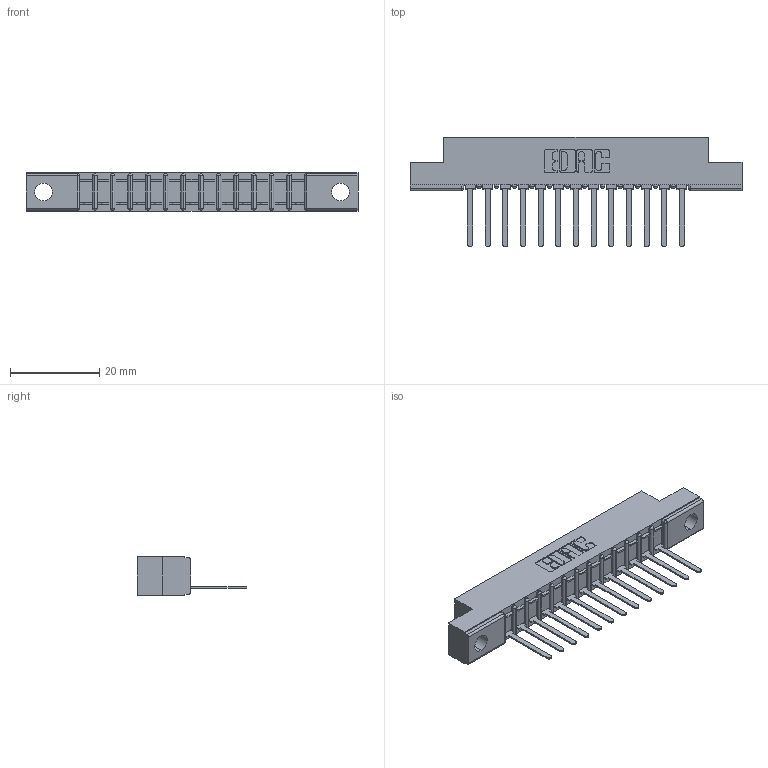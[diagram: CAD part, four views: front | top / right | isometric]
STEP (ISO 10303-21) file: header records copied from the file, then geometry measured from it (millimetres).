
FILE_DESCRIPTION (( 'STEP AP203' ), '1' );
FILE_NAME ('307-013-541-102.STEP', '2019-09-04T20:11:30', ( '' ), ( '' ), 'SwSTEP 2.0', 'SolidWorks 2016', '' );
FILE_SCHEMA (( 'CONFIG_CONTROL_DESIGN' ));
Length unit declared in the file: inch
Products named in the file (3): 307-013-541-102; 307 Part_.128 Dia Mounting Holes; 307-290-002_541
Assembly tree (14 placements, depth 2):
  307-013-541-102
    307 Part_.128 Dia Mounting Holes
    307-290-002_541  x13
Bounding box: 74.52 x 24.59 x 8.71 mm (x, y, z)
Volume: 4864 mm3; surface area: 8416.1 mm2
Topology: 14 solids, 14 shells, 1094 faces, 3339 edges, 2186 vertices
Faces by surface type: plane 655, cylinder 411, sphere 28
Entity records: 15440 total; most frequent: CARTESIAN_POINT 2600, ORIENTED_EDGE 2590, DIRECTION 2539, EDGE_CURVE 1295, VECTOR 977, LINE 977, VERTEX_POINT 842, AXIS2_PLACEMENT_3D 781
